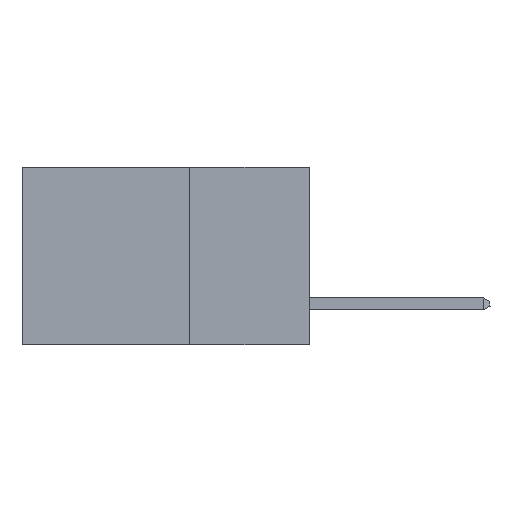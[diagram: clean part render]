
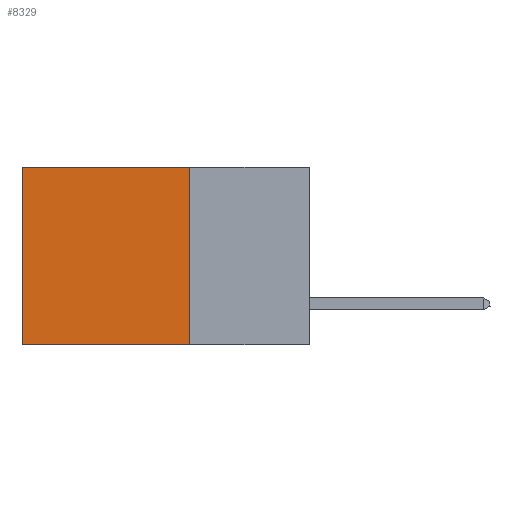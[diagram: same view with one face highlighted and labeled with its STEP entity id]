
A CAD part, left-side view. The second image highlights one B-rep face of the part: STEP entity #8329.
In plain terms, the highlighted planar face has unit normal (-1, 0, 0).
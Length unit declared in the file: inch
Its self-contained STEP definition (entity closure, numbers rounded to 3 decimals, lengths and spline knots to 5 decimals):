
#8 = ORIENTED_EDGE ( 'NONE', *, *, #69, .F. ) ;
#69 = EDGE_CURVE ( 'NONE', #5253, #536, #552, .T. ) ;
#267 = AXIS2_PLACEMENT_3D ( 'NONE', #7196, #13071, #11981 ) ;
#536 = VERTEX_POINT ( 'NONE', #13396 ) ;
#552 = LINE ( 'NONE', #9730, #5889 ) ;
#624 = DIRECTION ( 'NONE',  ( 0., 0., -1. ) ) ;
#737 = LINE ( 'NONE', #11585, #8244 ) ;
#1557 = VERTEX_POINT ( 'NONE', #7296 ) ;
#2168 = ORIENTED_EDGE ( 'NONE', *, *, #12507, .T. ) ;
#2743 = EDGE_CURVE ( 'NONE', #5253, #1557, #13276, .T. ) ;
#3812 = VERTEX_POINT ( 'NONE', #6222 ) ;
#5112 = LINE ( 'NONE', #11703, #7759 ) ;
#5253 = VERTEX_POINT ( 'NONE', #13048 ) ;
#5478 = ORIENTED_EDGE ( 'NONE', *, *, #2743, .T. ) ;
#5673 = EDGE_LOOP ( 'NONE', ( #2168, #9875, #8, #5478 ) ) ;
#5889 = VECTOR ( 'NONE', #624, 39.37008 ) ;
#6222 = CARTESIAN_POINT ( 'NONE',  ( 0.2875, 0.6, -0.37 ) ) ;
#7196 = CARTESIAN_POINT ( 'NONE',  ( 0.2875, 0.25, 0. ) ) ;
#7277 = VECTOR ( 'NONE', #11512, 39.37008 ) ;
#7296 = CARTESIAN_POINT ( 'NONE',  ( 0.2875, 0.6, 0. ) ) ;
#7759 = VECTOR ( 'NONE', #14050, 39.37008 ) ;
#8014 = FACE_OUTER_BOUND ( 'NONE', #5673, .T. ) ;
#8244 = VECTOR ( 'NONE', #13932, 39.37008 ) ;
#8329 = ADVANCED_FACE ( 'NONE', ( #8014 ), #12040, .F. ) ;
#9730 = CARTESIAN_POINT ( 'NONE',  ( 0.2875, 0.25, 0. ) ) ;
#9875 = ORIENTED_EDGE ( 'NONE', *, *, #12701, .F. ) ;
#11512 = DIRECTION ( 'NONE',  ( 0., 1., 0. ) ) ;
#11585 = CARTESIAN_POINT ( 'NONE',  ( 0.2875, 0.25, -0.37 ) ) ;
#11703 = CARTESIAN_POINT ( 'NONE',  ( 0.2875, 0.6, 0. ) ) ;
#11981 = DIRECTION ( 'NONE',  ( 0., 0., -1. ) ) ;
#12040 = PLANE ( 'NONE',  #267 ) ;
#12494 = CARTESIAN_POINT ( 'NONE',  ( 0.2875, 0.25, 0. ) ) ;
#12507 = EDGE_CURVE ( 'NONE', #1557, #3812, #5112, .T. ) ;
#12701 = EDGE_CURVE ( 'NONE', #536, #3812, #737, .T. ) ;
#13048 = CARTESIAN_POINT ( 'NONE',  ( 0.2875, 0.25, 0. ) ) ;
#13071 = DIRECTION ( 'NONE',  ( 1., 0., 0. ) ) ;
#13276 = LINE ( 'NONE', #12494, #7277 ) ;
#13396 = CARTESIAN_POINT ( 'NONE',  ( 0.2875, 0.25, -0.37 ) ) ;
#13932 = DIRECTION ( 'NONE',  ( 0., 1., 0. ) ) ;
#14050 = DIRECTION ( 'NONE',  ( 0., 0., -1. ) ) ;
